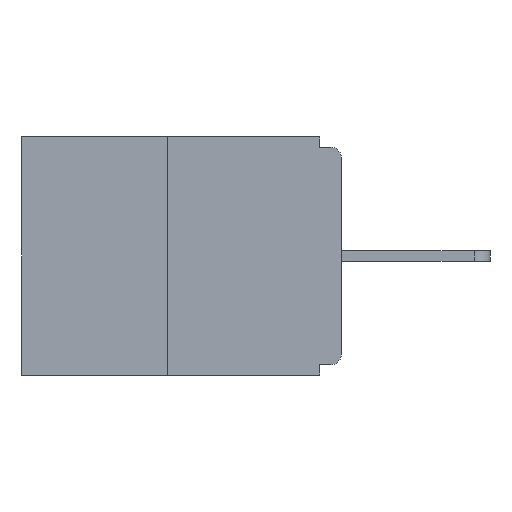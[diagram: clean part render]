
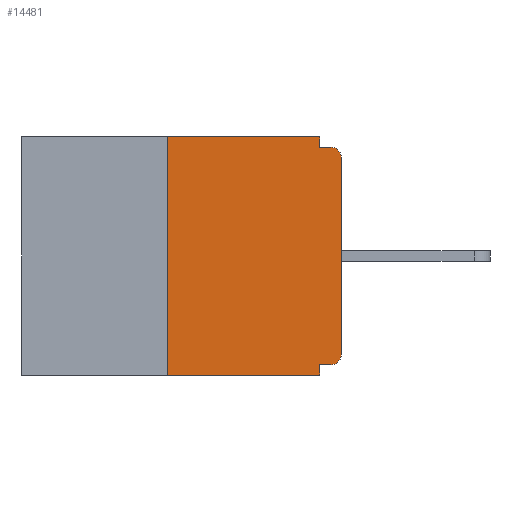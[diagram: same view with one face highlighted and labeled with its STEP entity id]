
A CAD part, left-side view. The second image highlights one B-rep face of the part: STEP entity #14481.
In plain terms, the highlighted planar face has unit normal (-1, 0, 0).
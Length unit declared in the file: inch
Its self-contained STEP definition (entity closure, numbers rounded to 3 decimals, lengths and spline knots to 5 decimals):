
#161 = ORIENTED_EDGE ( 'NONE', *, *, #13363, .T. ) ;
#232 = LINE ( 'NONE', #4732, #14320 ) ;
#327 = EDGE_CURVE ( 'NONE', #10367, #3317, #11589, .T. ) ;
#368 = CIRCLE ( 'NONE', #6669, 0.015 ) ;
#825 = ORIENTED_EDGE ( 'NONE', *, *, #16587, .F. ) ;
#889 = DIRECTION ( 'NONE',  ( -1., 0., 0. ) ) ;
#1031 = DIRECTION ( 'NONE',  ( 0., 0., -1. ) ) ;
#1206 = AXIS2_PLACEMENT_3D ( 'NONE', #12214, #4059, #13518 ) ;
#1247 = EDGE_CURVE ( 'NONE', #1734, #10367, #2363, .T. ) ;
#1265 = VERTEX_POINT ( 'NONE', #3602 ) ;
#1273 = ORIENTED_EDGE ( 'NONE', *, *, #5459, .F. ) ;
#1516 = DIRECTION ( 'NONE',  ( 0., 1., 0. ) ) ;
#1734 = VERTEX_POINT ( 'NONE', #9005 ) ;
#1935 = CARTESIAN_POINT ( 'NONE',  ( 0., 0.46, -0.343 ) ) ;
#2141 = LINE ( 'NONE', #2829, #9389 ) ;
#2227 = VERTEX_POINT ( 'NONE', #5463 ) ;
#2233 = DIRECTION ( 'NONE',  ( 0., 0., 1. ) ) ;
#2363 = LINE ( 'NONE', #15749, #13604 ) ;
#2829 = CARTESIAN_POINT ( 'NONE',  ( 0., 0.031, 0. ) ) ;
#3112 = CARTESIAN_POINT ( 'NONE',  ( 0., 0.031, -0.328 ) ) ;
#3317 = VERTEX_POINT ( 'NONE', #9010 ) ;
#3444 = VECTOR ( 'NONE', #15148, 39.37008 ) ;
#3469 = ORIENTED_EDGE ( 'NONE', *, *, #5096, .T. ) ;
#3602 = CARTESIAN_POINT ( 'NONE',  ( 0., 0., -0.03 ) ) ;
#3692 = VERTEX_POINT ( 'NONE', #11036 ) ;
#3909 = ORIENTED_EDGE ( 'NONE', *, *, #11536, .F. ) ;
#4059 = DIRECTION ( 'NONE',  ( -1., 0., 0. ) ) ;
#4732 = CARTESIAN_POINT ( 'NONE',  ( 0., 0., 0. ) ) ;
#5096 = EDGE_CURVE ( 'NONE', #7260, #1265, #232, .T. ) ;
#5111 = CIRCLE ( 'NONE', #1206, 0.015 ) ;
#5347 = LINE ( 'NONE', #1935, #5769 ) ;
#5459 = EDGE_CURVE ( 'NONE', #2227, #16041, #16287, .T. ) ;
#5463 = CARTESIAN_POINT ( 'NONE',  ( 0., 0.25, -0.343 ) ) ;
#5769 = VECTOR ( 'NONE', #10119, 39.37008 ) ;
#5785 = ORIENTED_EDGE ( 'NONE', *, *, #327, .F. ) ;
#6279 = AXIS2_PLACEMENT_3D ( 'NONE', #7837, #9237, #1031 ) ;
#6669 = AXIS2_PLACEMENT_3D ( 'NONE', #9091, #889, #10503 ) ;
#7028 = CARTESIAN_POINT ( 'NONE',  ( 0., 0.25, 0. ) ) ;
#7260 = VERTEX_POINT ( 'NONE', #13287 ) ;
#7438 = VECTOR ( 'NONE', #11256, 39.37008 ) ;
#7538 = VERTEX_POINT ( 'NONE', #13499 ) ;
#7837 = CARTESIAN_POINT ( 'NONE',  ( 0., 0.46, 0. ) ) ;
#8549 = ORIENTED_EDGE ( 'NONE', *, *, #11681, .T. ) ;
#9005 = CARTESIAN_POINT ( 'NONE',  ( 0., 0.015, -0.328 ) ) ;
#9010 = CARTESIAN_POINT ( 'NONE',  ( 0., 0.031, -0.343 ) ) ;
#9091 = CARTESIAN_POINT ( 'NONE',  ( 0., 0.015, -0.313 ) ) ;
#9237 = DIRECTION ( 'NONE',  ( 1., 0., 0. ) ) ;
#9389 = VECTOR ( 'NONE', #12366, 39.37008 ) ;
#9755 = DIRECTION ( 'NONE',  ( 0., -1., 0. ) ) ;
#9805 = CARTESIAN_POINT ( 'NONE',  ( 0., 0., -0.015 ) ) ;
#9841 = ORIENTED_EDGE ( 'NONE', *, *, #1247, .F. ) ;
#10119 = DIRECTION ( 'NONE',  ( 0., -1., 0. ) ) ;
#10367 = VERTEX_POINT ( 'NONE', #3112 ) ;
#10503 = DIRECTION ( 'NONE',  ( 0., 0., -1. ) ) ;
#10623 = EDGE_LOOP ( 'NONE', ( #825, #1273, #8549, #5785, #9841, #13431, #3469, #161, #3909, #11162 ) ) ;
#11036 = CARTESIAN_POINT ( 'NONE',  ( 0., 0.031, -0.015 ) ) ;
#11089 = DIRECTION ( 'NONE',  ( 0., 0., 1. ) ) ;
#11143 = LINE ( 'NONE', #9805, #3444 ) ;
#11162 = ORIENTED_EDGE ( 'NONE', *, *, #12092, .F. ) ;
#11233 = CARTESIAN_POINT ( 'NONE',  ( 0., 0.46, 0. ) ) ;
#11256 = DIRECTION ( 'NONE',  ( 0., 0., -1. ) ) ;
#11292 = EDGE_CURVE ( 'NONE', #1734, #7260, #368, .T. ) ;
#11519 = VECTOR ( 'NONE', #9755, 39.37008 ) ;
#11536 = EDGE_CURVE ( 'NONE', #3692, #17109, #11143, .T. ) ;
#11589 = LINE ( 'NONE', #14075, #7438 ) ;
#11681 = EDGE_CURVE ( 'NONE', #2227, #3317, #5347, .T. ) ;
#12092 = EDGE_CURVE ( 'NONE', #7538, #3692, #2141, .T. ) ;
#12214 = CARTESIAN_POINT ( 'NONE',  ( 0., 0.015, -0.03 ) ) ;
#12366 = DIRECTION ( 'NONE',  ( 0., 0., -1. ) ) ;
#13287 = CARTESIAN_POINT ( 'NONE',  ( 0., 0., -0.313 ) ) ;
#13363 = EDGE_CURVE ( 'NONE', #1265, #17109, #5111, .T. ) ;
#13431 = ORIENTED_EDGE ( 'NONE', *, *, #11292, .T. ) ;
#13499 = CARTESIAN_POINT ( 'NONE',  ( 0., 0.031, 0. ) ) ;
#13518 = DIRECTION ( 'NONE',  ( 0., 0., -1. ) ) ;
#13604 = VECTOR ( 'NONE', #1516, 39.37008 ) ;
#14075 = CARTESIAN_POINT ( 'NONE',  ( 0., 0.031, -0.343 ) ) ;
#14085 = LINE ( 'NONE', #11233, #11519 ) ;
#14320 = VECTOR ( 'NONE', #2233, 39.37008 ) ;
#14481 = ADVANCED_FACE ( 'NONE', ( #15144 ), #17113, .F. ) ;
#15144 = FACE_OUTER_BOUND ( 'NONE', #10623, .T. ) ;
#15148 = DIRECTION ( 'NONE',  ( 0., -1., 0. ) ) ;
#15478 = VECTOR ( 'NONE', #11089, 39.37008 ) ;
#15749 = CARTESIAN_POINT ( 'NONE',  ( 0., 0., -0.328 ) ) ;
#16041 = VERTEX_POINT ( 'NONE', #17445 ) ;
#16090 = CARTESIAN_POINT ( 'NONE',  ( 0., 0.015, -0.015 ) ) ;
#16287 = LINE ( 'NONE', #7028, #15478 ) ;
#16587 = EDGE_CURVE ( 'NONE', #16041, #7538, #14085, .T. ) ;
#17109 = VERTEX_POINT ( 'NONE', #16090 ) ;
#17113 = PLANE ( 'NONE',  #6279 ) ;
#17445 = CARTESIAN_POINT ( 'NONE',  ( 0., 0.25, 0. ) ) ;
